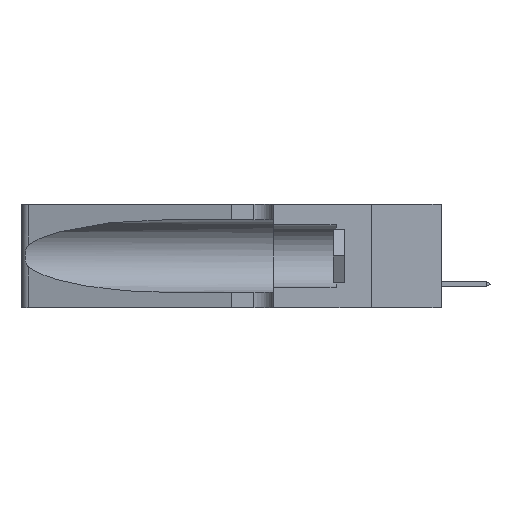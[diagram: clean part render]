
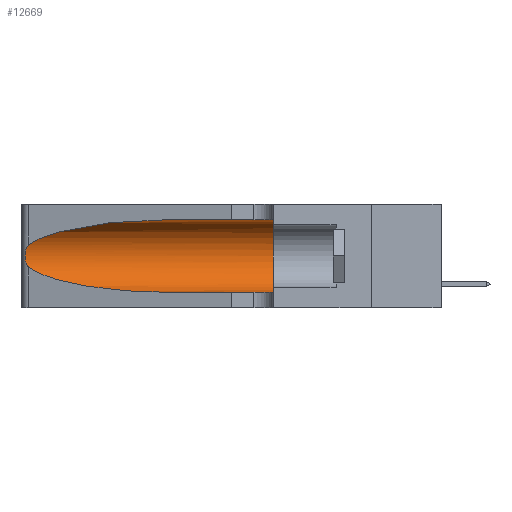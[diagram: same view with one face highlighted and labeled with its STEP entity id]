
A CAD part, left-side view. The second image highlights one B-rep face of the part: STEP entity #12669.
In plain terms, the highlighted cylindrical face has radius 3.308 mm (diameter 6.617 mm), a partial arc.
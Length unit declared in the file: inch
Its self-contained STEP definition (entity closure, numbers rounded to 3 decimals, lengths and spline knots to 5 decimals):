
#963 = VERTEX_POINT ( 'NONE', #15425 ) ;
#1086 = ORIENTED_EDGE ( 'NONE', *, *, #39233, .F. ) ;
#2872 = DIRECTION ( 'NONE',  ( 0., 0., -1. ) ) ;
#3122 = DIRECTION ( 'NONE',  ( 0., 1., 0. ) ) ;
#3149 = ORIENTED_EDGE ( 'NONE', *, *, #28075, .F. ) ;
#4170 = DIRECTION ( 'NONE',  ( 0., -1., 0. ) ) ;
#4636 = CARTESIAN_POINT ( 'NONE',  ( 0.25487, 1.22718, 0.22369 ) ) ;
#5171 = VECTOR ( 'NONE', #4170, 39.37008 ) ;
#5806 =( BOUNDED_CURVE ( )  B_SPLINE_CURVE ( 3, ( #10724, #22346, #23052, #23214 ),
 .UNSPECIFIED., .F., .F. ) 
 B_SPLINE_CURVE_WITH_KNOTS ( ( 4, 4 ),
 ( 3.44316, 4.71239 ),
 .UNSPECIFIED. ) 
 CURVE ( )  GEOMETRIC_REPRESENTATION_ITEM ( )  RATIONAL_B_SPLINE_CURVE ( ( 1., 0.87, 0.87, 1. ) ) 
 REPRESENTATION_ITEM ( '' )  );
#6489 =( BOUNDED_CURVE ( )  B_SPLINE_CURVE ( 3, ( #9152, #28676, #40805, #32278 ),
 .UNSPECIFIED., .F., .F. ) 
 B_SPLINE_CURVE_WITH_KNOTS ( ( 4, 4 ),
 ( 1.5708, 2.84003 ),
 .UNSPECIFIED. ) 
 CURVE ( )  GEOMETRIC_REPRESENTATION_ITEM ( )  RATIONAL_B_SPLINE_CURVE ( ( 1., 0.87, 0.87, 1. ) ) 
 REPRESENTATION_ITEM ( '' )  );
#7905 = ORIENTED_EDGE ( 'NONE', *, *, #8176, .T. ) ;
#8176 = EDGE_CURVE ( 'NONE', #8394, #31889, #5806, .T. ) ;
#8389 = CARTESIAN_POINT ( 'NONE',  ( 0.26075, 1.23896, 0.19203 ) ) ;
#8394 = VERTEX_POINT ( 'NONE', #14312 ) ;
#8796 = CIRCLE ( 'NONE', #34667, 0.13025 ) ;
#9152 = CARTESIAN_POINT ( 'NONE',  ( 0.1305, 0.72297, 0.31525 ) ) ;
#10724 = CARTESIAN_POINT ( 'NONE',  ( 0.25487, 1.22718, 0.14631 ) ) ;
#12324 = CARTESIAN_POINT ( 'NONE',  ( 0.26017, 1.23833, 0.17102 ) ) ;
#12669 = ADVANCED_FACE ( 'NONE', ( #42788 ), #14664, .F. ) ;
#14312 = CARTESIAN_POINT ( 'NONE',  ( 0.25487, 1.22718, 0.14631 ) ) ;
#14664 = CYLINDRICAL_SURFACE ( 'NONE', #44488, 0.13025 ) ;
#15425 = CARTESIAN_POINT ( 'NONE',  ( 0.25487, 1.22718, 0.22369 ) ) ;
#16356 = CARTESIAN_POINT ( 'NONE',  ( 0.1305, 1.61858, 0.05475 ) ) ;
#16707 = CARTESIAN_POINT ( 'NONE',  ( 0.26075, 1.23896, 0.178 ) ) ;
#16883 = CARTESIAN_POINT ( 'NONE',  ( 0.1305, 1.61858, 0.31525 ) ) ;
#17182 = EDGE_CURVE ( 'NONE', #31889, #30671, #39458, .T. ) ;
#17674 = DIRECTION ( 'NONE',  ( 0., -1., 0. ) ) ;
#18003 = VECTOR ( 'NONE', #28733, 39.37008 ) ;
#20327 = CARTESIAN_POINT ( 'NONE',  ( 0.25639, 1.23184, 0.21858 ) ) ;
#20648 = CARTESIAN_POINT ( 'NONE',  ( 0.25789, 1.23486, 0.15765 ) ) ;
#21431 = VERTEX_POINT ( 'NONE', #45664 ) ;
#22334 = ORIENTED_EDGE ( 'NONE', *, *, #17182, .T. ) ;
#22346 = CARTESIAN_POINT ( 'NONE',  ( 0.2373, 1.15595, 0.08982 ) ) ;
#23052 = CARTESIAN_POINT ( 'NONE',  ( 0.18966, 0.96281, 0.05475 ) ) ;
#23214 = CARTESIAN_POINT ( 'NONE',  ( 0.1305, 0.72297, 0.05475 ) ) ;
#24306 = CARTESIAN_POINT ( 'NONE',  ( 0.25555, 1.22993, 0.14849 ) ) ;
#24571 = ORIENTED_EDGE ( 'NONE', *, *, #47824, .T. ) ;
#25402 = CARTESIAN_POINT ( 'NONE',  ( 0.1305, 0.72297, 0.05475 ) ) ;
#26539 = CARTESIAN_POINT ( 'NONE',  ( 0.1305, 0.35, 0.185 ) ) ;
#27747 = VERTEX_POINT ( 'NONE', #37939 ) ;
#27815 = ORIENTED_EDGE ( 'NONE', *, *, #45088, .T. ) ;
#28075 = EDGE_CURVE ( 'NONE', #27747, #21431, #39987, .T. ) ;
#28216 = CARTESIAN_POINT ( 'NONE',  ( 0.25854, 1.2359, 0.20912 ) ) ;
#28676 = CARTESIAN_POINT ( 'NONE',  ( 0.18966, 0.96281, 0.31525 ) ) ;
#28733 = DIRECTION ( 'NONE',  ( 0., -1., 0. ) ) ;
#30671 = VERTEX_POINT ( 'NONE', #37981 ) ;
#31889 = VERTEX_POINT ( 'NONE', #25402 ) ;
#32278 = CARTESIAN_POINT ( 'NONE',  ( 0.25487, 1.22718, 0.22369 ) ) ;
#33613 = CARTESIAN_POINT ( 'NONE',  ( 0.1305, 1.61858, 0.185 ) ) ;
#34575 = DIRECTION ( 'NONE',  ( 0., 0., 1. ) ) ;
#34667 = AXIS2_PLACEMENT_3D ( 'NONE', #26539, #3122, #34575 ) ;
#35741 = CARTESIAN_POINT ( 'NONE',  ( 0.25787, 1.23484, 0.2124 ) ) ;
#36241 = CARTESIAN_POINT ( 'NONE',  ( 0.26018, 1.23835, 0.19895 ) ) ;
#37939 = CARTESIAN_POINT ( 'NONE',  ( 0.1305, 0.72297, 0.31525 ) ) ;
#37981 = CARTESIAN_POINT ( 'NONE',  ( 0.1305, 0.35, 0.05475 ) ) ;
#39233 = EDGE_CURVE ( 'NONE', #21431, #30671, #8796, .T. ) ;
#39458 = LINE ( 'NONE', #16356, #5171 ) ;
#39696 = CARTESIAN_POINT ( 'NONE',  ( 0.25639, 1.23186, 0.15144 ) ) ;
#39987 = LINE ( 'NONE', #16883, #18003 ) ;
#40344 = CARTESIAN_POINT ( 'NONE',  ( 0.25856, 1.23593, 0.16098 ) ) ;
#40805 = CARTESIAN_POINT ( 'NONE',  ( 0.2373, 1.15595, 0.28018 ) ) ;
#42788 = FACE_OUTER_BOUND ( 'NONE', #43690, .T. ) ;
#43690 = EDGE_LOOP ( 'NONE', ( #27815, #24571, #7905, #22334, #1086, #3149 ) ) ;
#43719 = CARTESIAN_POINT ( 'NONE',  ( 0.25555, 1.22994, 0.2215 ) ) ;
#44488 = AXIS2_PLACEMENT_3D ( 'NONE', #33613, #17674, #2872 ) ;
#45088 = EDGE_CURVE ( 'NONE', #27747, #963, #6489, .T. ) ;
#45664 = CARTESIAN_POINT ( 'NONE',  ( 0.1305, 0.35, 0.31525 ) ) ;
#47403 = B_SPLINE_CURVE_WITH_KNOTS ( 'NONE', 3,
 ( #4636, #43719, #20327, #35741, #28216, #36241, #8389, #16707, #12324, #40344, #20648, #39696, #24306, #47938 ),
 .UNSPECIFIED., .F., .F.,
 ( 4, 2, 2, 2, 2, 2, 4 ),
 ( 0., 0.00027, 0.00053, 0.00107, 0.0016, 0.00187, 0.00214 ),
 .UNSPECIFIED. ) ;
#47824 = EDGE_CURVE ( 'NONE', #963, #8394, #47403, .T. ) ;
#47938 = CARTESIAN_POINT ( 'NONE',  ( 0.25487, 1.22718, 0.14631 ) ) ;
